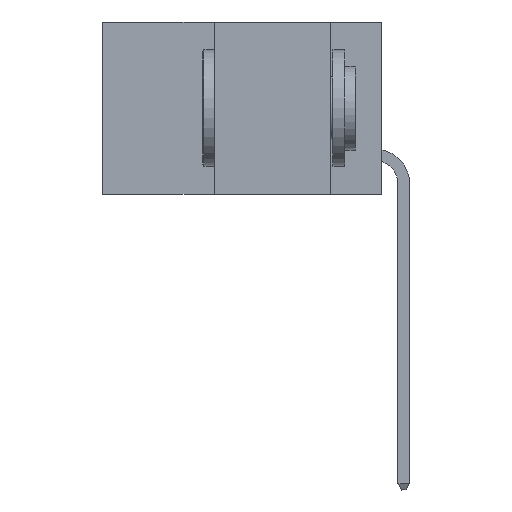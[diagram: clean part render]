
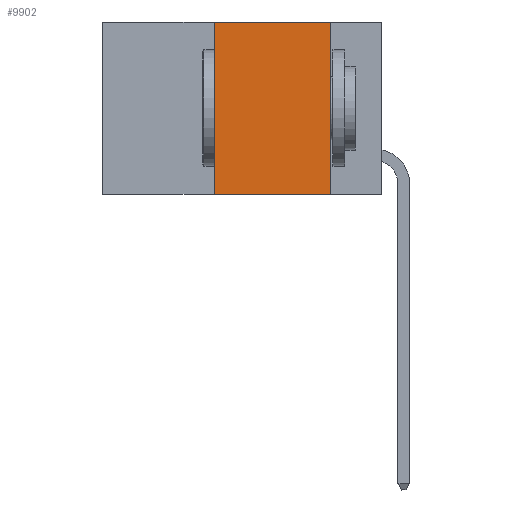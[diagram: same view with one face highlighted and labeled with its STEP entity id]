
A CAD part, left-side view. The second image highlights one B-rep face of the part: STEP entity #9902.
In plain terms, the highlighted planar face has unit normal (-1, 0, 0).
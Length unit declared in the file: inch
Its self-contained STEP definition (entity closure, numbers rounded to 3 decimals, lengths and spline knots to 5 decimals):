
#182 = ORIENTED_EDGE ( 'NONE', *, *, #6409, .T. ) ;
#265 = EDGE_CURVE ( 'NONE', #5674, #2153, #829, .T. ) ;
#829 = LINE ( 'NONE', #2813, #3867 ) ;
#957 = CARTESIAN_POINT ( 'NONE',  ( 0., 0.6, 0. ) ) ;
#1294 = CARTESIAN_POINT ( 'NONE',  ( 0., 0.11, -0.37 ) ) ;
#1336 = DIRECTION ( 'NONE',  ( 0., -1., 0. ) ) ;
#1352 = AXIS2_PLACEMENT_3D ( 'NONE', #5300, #7167, #3625 ) ;
#1921 = CARTESIAN_POINT ( 'NONE',  ( 0., 0.36, 0. ) ) ;
#1985 = CARTESIAN_POINT ( 'NONE',  ( 0., 0.36, 0. ) ) ;
#2061 = DIRECTION ( 'NONE',  ( 0., 0., 1. ) ) ;
#2153 = VERTEX_POINT ( 'NONE', #1294 ) ;
#2476 = ORIENTED_EDGE ( 'NONE', *, *, #7766, .F. ) ;
#2556 = VECTOR ( 'NONE', #8859, 39.37008 ) ;
#2717 = LINE ( 'NONE', #5743, #5736 ) ;
#2813 = CARTESIAN_POINT ( 'NONE',  ( 0., 0.11, 0. ) ) ;
#3067 = VERTEX_POINT ( 'NONE', #1921 ) ;
#3625 = DIRECTION ( 'NONE',  ( 0., 0., -1. ) ) ;
#3867 = VECTOR ( 'NONE', #6473, 39.37008 ) ;
#5300 = CARTESIAN_POINT ( 'NONE',  ( 0., 0.6, 0. ) ) ;
#5674 = VERTEX_POINT ( 'NONE', #6961 ) ;
#5736 = VECTOR ( 'NONE', #1336, 39.37008 ) ;
#5743 = CARTESIAN_POINT ( 'NONE',  ( 0., 0.6, -0.37 ) ) ;
#6409 = EDGE_CURVE ( 'NONE', #11104, #2153, #2717, .T. ) ;
#6473 = DIRECTION ( 'NONE',  ( 0., 0., -1. ) ) ;
#6961 = CARTESIAN_POINT ( 'NONE',  ( 0., 0.11, 0. ) ) ;
#7098 = ORIENTED_EDGE ( 'NONE', *, *, #265, .F. ) ;
#7167 = DIRECTION ( 'NONE',  ( 1., 0., 0. ) ) ;
#7766 = EDGE_CURVE ( 'NONE', #11104, #3067, #9350, .T. ) ;
#7977 = LINE ( 'NONE', #957, #2556 ) ;
#8250 = ORIENTED_EDGE ( 'NONE', *, *, #8849, .F. ) ;
#8849 = EDGE_CURVE ( 'NONE', #3067, #5674, #7977, .T. ) ;
#8859 = DIRECTION ( 'NONE',  ( 0., -1., 0. ) ) ;
#9085 = VECTOR ( 'NONE', #2061, 39.37008 ) ;
#9350 = LINE ( 'NONE', #1985, #9085 ) ;
#9902 = ADVANCED_FACE ( 'NONE', ( #10571 ), #10624, .F. ) ;
#9940 = CARTESIAN_POINT ( 'NONE',  ( 0., 0.36, -0.37 ) ) ;
#10571 = FACE_OUTER_BOUND ( 'NONE', #10592, .T. ) ;
#10592 = EDGE_LOOP ( 'NONE', ( #7098, #8250, #2476, #182 ) ) ;
#10624 = PLANE ( 'NONE',  #1352 ) ;
#11104 = VERTEX_POINT ( 'NONE', #9940 ) ;
